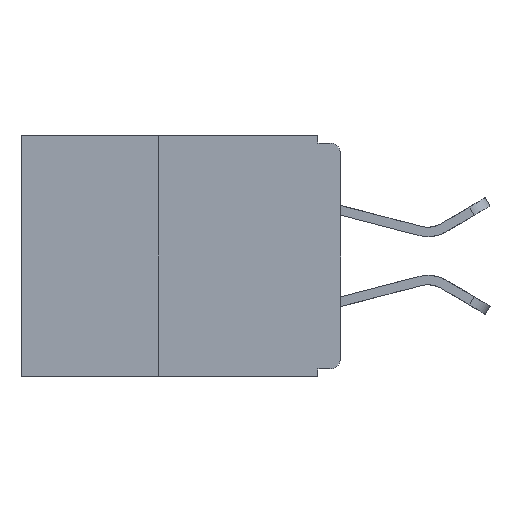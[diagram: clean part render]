
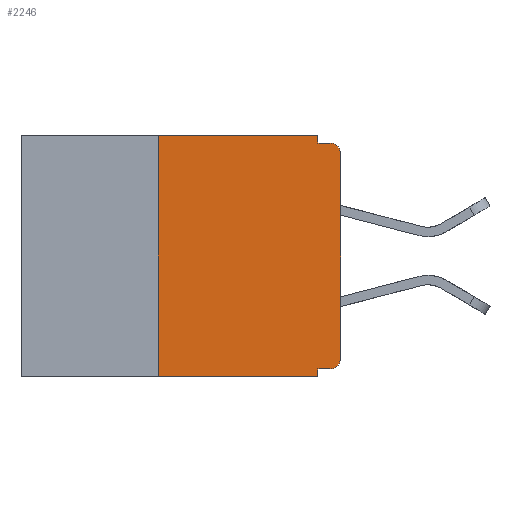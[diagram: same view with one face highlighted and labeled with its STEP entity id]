
A CAD part, left-side view. The second image highlights one B-rep face of the part: STEP entity #2246.
In plain terms, the highlighted planar face has unit normal (-1, 0, 0).
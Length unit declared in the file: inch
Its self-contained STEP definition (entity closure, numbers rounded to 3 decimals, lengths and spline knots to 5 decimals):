
#108 = VECTOR ( 'NONE', #10503, 39.37008 ) ;
#199 = DIRECTION ( 'NONE',  ( 0., 0., -1. ) ) ;
#318 = VECTOR ( 'NONE', #5170, 39.37008 ) ;
#361 = LINE ( 'NONE', #4034, #12722 ) ;
#1266 = EDGE_CURVE ( 'NONE', #8917, #13797, #5696, .T. ) ;
#1786 = AXIS2_PLACEMENT_3D ( 'NONE', #5120, #16590, #6841 ) ;
#1819 = VECTOR ( 'NONE', #199, 39.37008 ) ;
#2246 = ADVANCED_FACE ( 'NONE', ( #14199 ), #15132, .F. ) ;
#2451 = LINE ( 'NONE', #7045, #6485 ) ;
#2488 = CARTESIAN_POINT ( 'NONE',  ( 0., 0.015, -0.01 ) ) ;
#2761 = EDGE_CURVE ( 'NONE', #15163, #7945, #9300, .T. ) ;
#3066 = VERTEX_POINT ( 'NONE', #13671 ) ;
#3414 = ORIENTED_EDGE ( 'NONE', *, *, #2761, .F. ) ;
#4034 = CARTESIAN_POINT ( 'NONE',  ( 0., 0.437, 0. ) ) ;
#4209 = VERTEX_POINT ( 'NONE', #9182 ) ;
#4407 = VERTEX_POINT ( 'NONE', #4614 ) ;
#4614 = CARTESIAN_POINT ( 'NONE',  ( 0., 0.031, -0.33 ) ) ;
#4987 = CIRCLE ( 'NONE', #1786, 0.015 ) ;
#5097 = CARTESIAN_POINT ( 'NONE',  ( 0., 0., -0.32 ) ) ;
#5120 = CARTESIAN_POINT ( 'NONE',  ( 0., 0.015, -0.305 ) ) ;
#5170 = DIRECTION ( 'NONE',  ( 0., 1., 0. ) ) ;
#5269 = ORIENTED_EDGE ( 'NONE', *, *, #14086, .F. ) ;
#5314 = DIRECTION ( 'NONE',  ( -1., 0., 0. ) ) ;
#5322 = VERTEX_POINT ( 'NONE', #11952 ) ;
#5696 = CIRCLE ( 'NONE', #5911, 0.015 ) ;
#5747 = DIRECTION ( 'NONE',  ( 0., 0., -1. ) ) ;
#5771 = DIRECTION ( 'NONE',  ( 0., -1., 0. ) ) ;
#5911 = AXIS2_PLACEMENT_3D ( 'NONE', #7787, #5314, #5747 ) ;
#6082 = CARTESIAN_POINT ( 'NONE',  ( 0., 0.031, -0.01 ) ) ;
#6254 = ORIENTED_EDGE ( 'NONE', *, *, #15906, .T. ) ;
#6485 = VECTOR ( 'NONE', #13600, 39.37008 ) ;
#6806 = ORIENTED_EDGE ( 'NONE', *, *, #9090, .F. ) ;
#6841 = DIRECTION ( 'NONE',  ( 0., 0., -1. ) ) ;
#7045 = CARTESIAN_POINT ( 'NONE',  ( 0., 0.437, -0.33 ) ) ;
#7190 = CARTESIAN_POINT ( 'NONE',  ( 0., 0., 0. ) ) ;
#7787 = CARTESIAN_POINT ( 'NONE',  ( 0., 0.015, -0.025 ) ) ;
#7945 = VERTEX_POINT ( 'NONE', #14593 ) ;
#8420 = VERTEX_POINT ( 'NONE', #6082 ) ;
#8833 = DIRECTION ( 'NONE',  ( 0., -1., 0. ) ) ;
#8917 = VERTEX_POINT ( 'NONE', #18701 ) ;
#9090 = EDGE_CURVE ( 'NONE', #4209, #8420, #19271, .T. ) ;
#9182 = CARTESIAN_POINT ( 'NONE',  ( 0., 0.031, 0. ) ) ;
#9300 = LINE ( 'NONE', #5097, #318 ) ;
#9509 = DIRECTION ( 'NONE',  ( 0., 0., -1. ) ) ;
#9524 = DIRECTION ( 'NONE',  ( 0., 0., 1. ) ) ;
#9708 = EDGE_LOOP ( 'NONE', ( #20399, #20664, #19469, #6806, #12239, #19743, #19031, #5269, #3414, #6254 ) ) ;
#10503 = DIRECTION ( 'NONE',  ( 0., 0., 1. ) ) ;
#11458 = EDGE_CURVE ( 'NONE', #5322, #4407, #2451, .T. ) ;
#11946 = CARTESIAN_POINT ( 'NONE',  ( 0., 0.031, -0.33 ) ) ;
#11952 = CARTESIAN_POINT ( 'NONE',  ( 0., 0.25, -0.33 ) ) ;
#12239 = ORIENTED_EDGE ( 'NONE', *, *, #20536, .F. ) ;
#12722 = VECTOR ( 'NONE', #5771, 39.37008 ) ;
#13089 = VERTEX_POINT ( 'NONE', #20216 ) ;
#13600 = DIRECTION ( 'NONE',  ( 0., -1., 0. ) ) ;
#13671 = CARTESIAN_POINT ( 'NONE',  ( 0., 0.25, 0. ) ) ;
#13797 = VERTEX_POINT ( 'NONE', #2488 ) ;
#14086 = EDGE_CURVE ( 'NONE', #7945, #4407, #19336, .T. ) ;
#14199 = FACE_OUTER_BOUND ( 'NONE', #9708, .T. ) ;
#14321 = DIRECTION ( 'NONE',  ( 0., 0., -1. ) ) ;
#14345 = DIRECTION ( 'NONE',  ( 1., 0., 0. ) ) ;
#14593 = CARTESIAN_POINT ( 'NONE',  ( 0., 0.031, -0.32 ) ) ;
#14686 = CARTESIAN_POINT ( 'NONE',  ( 0., 0.015, -0.32 ) ) ;
#14692 = CARTESIAN_POINT ( 'NONE',  ( 0., 0.437, 0. ) ) ;
#15132 = PLANE ( 'NONE',  #18870 ) ;
#15163 = VERTEX_POINT ( 'NONE', #14686 ) ;
#15906 = EDGE_CURVE ( 'NONE', #15163, #13089, #4987, .T. ) ;
#15942 = VECTOR ( 'NONE', #8833, 39.37008 ) ;
#16590 = DIRECTION ( 'NONE',  ( -1., 0., 0. ) ) ;
#16902 = EDGE_CURVE ( 'NONE', #5322, #3066, #17738, .T. ) ;
#17581 = CARTESIAN_POINT ( 'NONE',  ( 0., 0.031, 0. ) ) ;
#17701 = LINE ( 'NONE', #7190, #108 ) ;
#17738 = LINE ( 'NONE', #20758, #18248 ) ;
#17868 = EDGE_CURVE ( 'NONE', #13089, #8917, #17701, .T. ) ;
#18248 = VECTOR ( 'NONE', #9524, 39.37008 ) ;
#18492 = CARTESIAN_POINT ( 'NONE',  ( 0., 0., -0.01 ) ) ;
#18701 = CARTESIAN_POINT ( 'NONE',  ( 0., 0., -0.025 ) ) ;
#18870 = AXIS2_PLACEMENT_3D ( 'NONE', #14692, #14345, #14321 ) ;
#19031 = ORIENTED_EDGE ( 'NONE', *, *, #11458, .T. ) ;
#19271 = LINE ( 'NONE', #17581, #20733 ) ;
#19336 = LINE ( 'NONE', #11946, #1819 ) ;
#19469 = ORIENTED_EDGE ( 'NONE', *, *, #21029, .F. ) ;
#19743 = ORIENTED_EDGE ( 'NONE', *, *, #16902, .F. ) ;
#20143 = LINE ( 'NONE', #18492, #15942 ) ;
#20216 = CARTESIAN_POINT ( 'NONE',  ( 0., 0., -0.305 ) ) ;
#20399 = ORIENTED_EDGE ( 'NONE', *, *, #17868, .T. ) ;
#20536 = EDGE_CURVE ( 'NONE', #3066, #4209, #361, .T. ) ;
#20664 = ORIENTED_EDGE ( 'NONE', *, *, #1266, .T. ) ;
#20733 = VECTOR ( 'NONE', #9509, 39.37008 ) ;
#20758 = CARTESIAN_POINT ( 'NONE',  ( 0., 0.25, -0.33 ) ) ;
#21029 = EDGE_CURVE ( 'NONE', #8420, #13797, #20143, .T. ) ;
